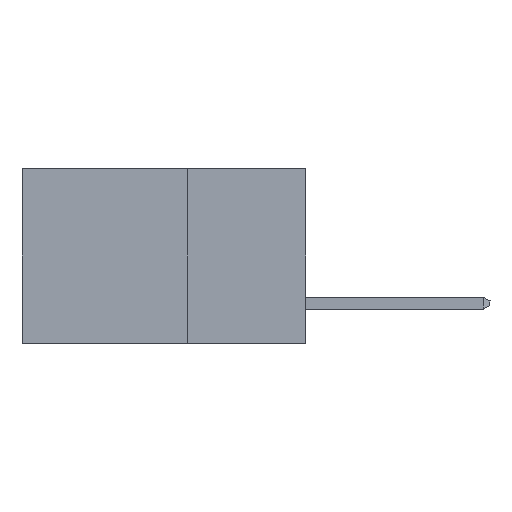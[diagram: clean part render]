
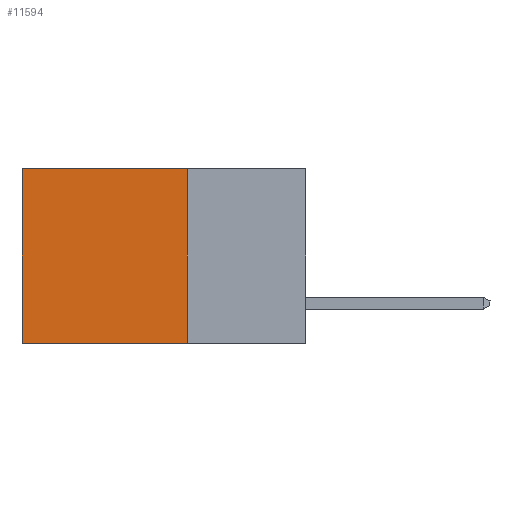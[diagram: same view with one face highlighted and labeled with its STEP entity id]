
A CAD part, left-side view. The second image highlights one B-rep face of the part: STEP entity #11594.
In plain terms, the highlighted planar face has unit normal (-1, 0, 0).
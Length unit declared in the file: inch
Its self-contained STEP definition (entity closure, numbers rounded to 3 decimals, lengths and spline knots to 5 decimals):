
#42 = CARTESIAN_POINT ( 'NONE',  ( 0.298, 0.25, 0. ) ) ;
#114 = DIRECTION ( 'NONE',  ( 1., 0., 0. ) ) ;
#1585 = LINE ( 'NONE', #15957, #15243 ) ;
#2072 = DIRECTION ( 'NONE',  ( 0., 1., 0. ) ) ;
#3122 = VERTEX_POINT ( 'NONE', #9958 ) ;
#3488 = CARTESIAN_POINT ( 'NONE',  ( 0.298, 0.25, -0.37 ) ) ;
#6161 = VECTOR ( 'NONE', #15183, 39.37008 ) ;
#6497 = LINE ( 'NONE', #7178, #15240 ) ;
#7178 = CARTESIAN_POINT ( 'NONE',  ( 0.298, 0.25, 0. ) ) ;
#7874 = ORIENTED_EDGE ( 'NONE', *, *, #10318, .T. ) ;
#7883 = PLANE ( 'NONE',  #16801 ) ;
#7894 = LINE ( 'NONE', #11120, #6161 ) ;
#8013 = VERTEX_POINT ( 'NONE', #11371 ) ;
#8222 = DIRECTION ( 'NONE',  ( 0., 1., 0. ) ) ;
#8697 = EDGE_CURVE ( 'NONE', #8013, #3122, #1585, .T. ) ;
#9958 = CARTESIAN_POINT ( 'NONE',  ( 0.298, 0.25, -0.37 ) ) ;
#10106 = LINE ( 'NONE', #3488, #10571 ) ;
#10259 = DIRECTION ( 'NONE',  ( 0., 0., -1. ) ) ;
#10302 = CARTESIAN_POINT ( 'NONE',  ( 0.298, 0.6, -0.37 ) ) ;
#10318 = EDGE_CURVE ( 'NONE', #12438, #10575, #7894, .T. ) ;
#10571 = VECTOR ( 'NONE', #8222, 39.37008 ) ;
#10575 = VERTEX_POINT ( 'NONE', #10302 ) ;
#11120 = CARTESIAN_POINT ( 'NONE',  ( 0.298, 0.6, 0. ) ) ;
#11371 = CARTESIAN_POINT ( 'NONE',  ( 0.298, 0.25, 0. ) ) ;
#11594 = ADVANCED_FACE ( 'NONE', ( #11956 ), #7883, .F. ) ;
#11956 = FACE_OUTER_BOUND ( 'NONE', #13983, .T. ) ;
#12233 = CARTESIAN_POINT ( 'NONE',  ( 0.298, 0.6, 0. ) ) ;
#12438 = VERTEX_POINT ( 'NONE', #12233 ) ;
#13983 = EDGE_LOOP ( 'NONE', ( #7874, #19748, #18373, #14741 ) ) ;
#14100 = EDGE_CURVE ( 'NONE', #8013, #12438, #6497, .T. ) ;
#14741 = ORIENTED_EDGE ( 'NONE', *, *, #14100, .T. ) ;
#15183 = DIRECTION ( 'NONE',  ( 0., 0., -1. ) ) ;
#15240 = VECTOR ( 'NONE', #2072, 39.37008 ) ;
#15243 = VECTOR ( 'NONE', #10259, 39.37008 ) ;
#15338 = DIRECTION ( 'NONE',  ( 0., 0., -1. ) ) ;
#15904 = EDGE_CURVE ( 'NONE', #3122, #10575, #10106, .T. ) ;
#15957 = CARTESIAN_POINT ( 'NONE',  ( 0.298, 0.25, 0. ) ) ;
#16801 = AXIS2_PLACEMENT_3D ( 'NONE', #42, #114, #15338 ) ;
#18373 = ORIENTED_EDGE ( 'NONE', *, *, #8697, .F. ) ;
#19748 = ORIENTED_EDGE ( 'NONE', *, *, #15904, .F. ) ;
